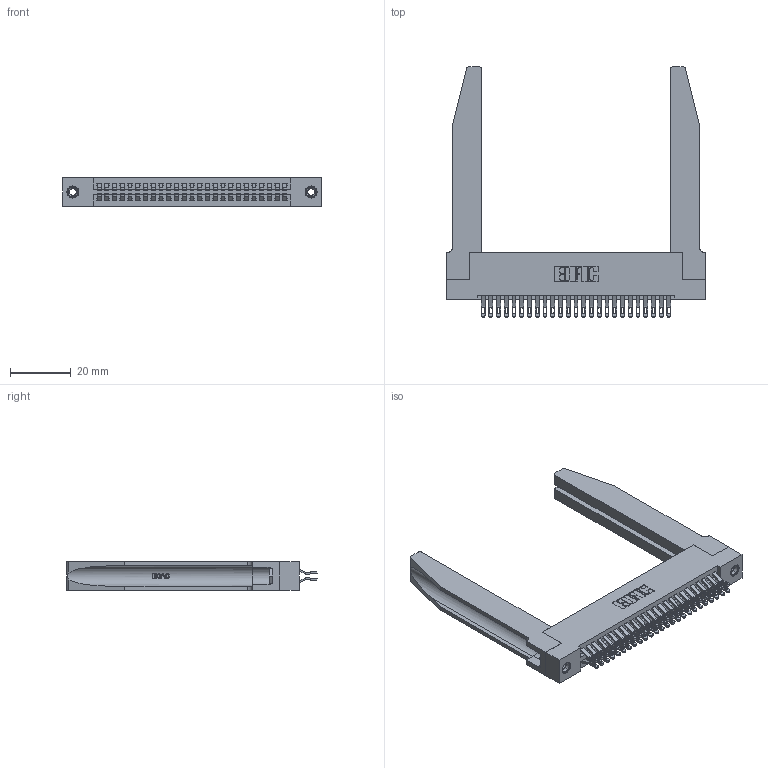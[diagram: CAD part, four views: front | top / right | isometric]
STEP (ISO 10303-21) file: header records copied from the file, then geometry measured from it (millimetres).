
FILE_DESCRIPTION (( 'STEP AP203' ), '1' );
FILE_NAME ('345-050-555-278.STEP', '2019-10-29T12:46:25', ( '' ), ( '' ), 'SwSTEP 2.0', 'SolidWorks 2016', '' );
FILE_SCHEMA (( 'CONFIG_CONTROL_DESIGN' ));
Length unit declared in the file: inch
Products named in the file (5): 345-050-555-278; 345-292-001_555 Tail; 345-220-078_345-220-078; 345 Part_Flush Mounting Lugs - 0.156 Dia-TH; 345-250-001_345-250-001-102
Assembly tree (55 placements, depth 2):
  345-050-555-278
    345 Part_Flush Mounting Lugs - 0.156 Dia-TH
    345-292-001_555 Tail  x50
    345-250-001_345-250-001-102  x2
    345-220-078_345-220-078  x2
Bounding box: 84.73 x 82.09 x 9.4 mm (x, y, z)
Volume: 15988.8 mm3; surface area: 19161.8 mm2
Topology: 55 solids, 55 shells, 3160 faces, 9799 edges, 6522 vertices
Faces by surface type: plane 1772, cylinder 1336, bspline 36, cone 12, torus 4
Entity records: 26970 total; most frequent: CARTESIAN_POINT 5489, ORIENTED_EDGE 4290, DIRECTION 3823, EDGE_CURVE 2145, VECTOR 1799, LINE 1799, VERTEX_POINT 1424, AXIS2_PLACEMENT_3D 1012
